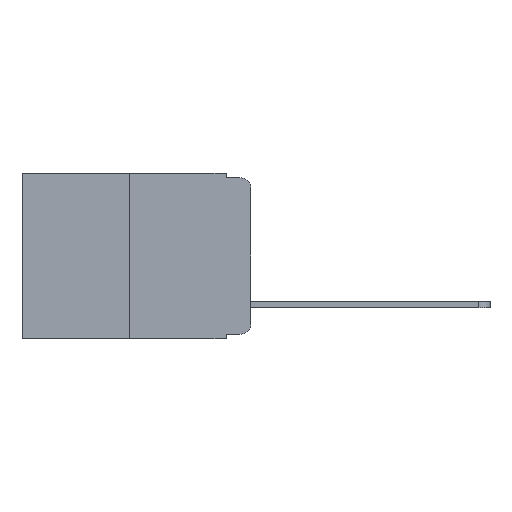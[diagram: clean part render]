
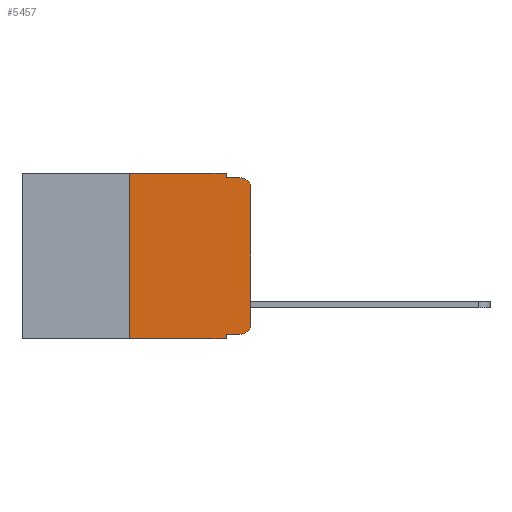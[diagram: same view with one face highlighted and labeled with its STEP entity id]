
A CAD part, left-side view. The second image highlights one B-rep face of the part: STEP entity #5457.
In plain terms, the highlighted planar face has unit normal (-1, 0, 0).
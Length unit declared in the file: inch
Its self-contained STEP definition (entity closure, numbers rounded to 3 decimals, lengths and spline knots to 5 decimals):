
#1 = VERTEX_POINT ( 'NONE', #9375 ) ;
#126 = DIRECTION ( 'NONE',  ( 0., 0., -1. ) ) ;
#350 = ORIENTED_EDGE ( 'NONE', *, *, #6454, .F. ) ;
#742 = VERTEX_POINT ( 'NONE', #3904 ) ;
#983 = DIRECTION ( 'NONE',  ( 0., 0., 1. ) ) ;
#1286 = ORIENTED_EDGE ( 'NONE', *, *, #6357, .T. ) ;
#1428 = DIRECTION ( 'NONE',  ( 0., 0., -1. ) ) ;
#1685 = LINE ( 'NONE', #3906, #8695 ) ;
#1980 = LINE ( 'NONE', #2163, #4214 ) ;
#2163 = CARTESIAN_POINT ( 'NONE',  ( 0., 0.051, -0.01 ) ) ;
#2404 = DIRECTION ( 'NONE',  ( 1., 0., 0. ) ) ;
#2427 = ORIENTED_EDGE ( 'NONE', *, *, #2499, .F. ) ;
#2429 = EDGE_CURVE ( 'NONE', #742, #3258, #10871, .T. ) ;
#2499 = EDGE_CURVE ( 'NONE', #16361, #14265, #15868, .T. ) ;
#2777 = VECTOR ( 'NONE', #983, 39.37008 ) ;
#3258 = VERTEX_POINT ( 'NONE', #6796 ) ;
#3377 = EDGE_CURVE ( 'NONE', #7624, #3258, #1980, .T. ) ;
#3547 = LINE ( 'NONE', #13163, #12404 ) ;
#3613 = AXIS2_PLACEMENT_3D ( 'NONE', #10280, #2404, #11426 ) ;
#3671 = PLANE ( 'NONE',  #3613 ) ;
#3904 = CARTESIAN_POINT ( 'NONE',  ( 0., 0., -0.03 ) ) ;
#3906 = CARTESIAN_POINT ( 'NONE',  ( 0., 0.25, 0. ) ) ;
#4214 = VECTOR ( 'NONE', #8501, 39.37008 ) ;
#4229 = FACE_OUTER_BOUND ( 'NONE', #7039, .T. ) ;
#4566 = CARTESIAN_POINT ( 'NONE',  ( 0., 0.02, -0.333 ) ) ;
#4628 = DIRECTION ( 'NONE',  ( 0., -1., 0. ) ) ;
#4681 = CARTESIAN_POINT ( 'NONE',  ( 0., 0.473, -0.343 ) ) ;
#4726 = ORIENTED_EDGE ( 'NONE', *, *, #2429, .T. ) ;
#5040 = CARTESIAN_POINT ( 'NONE',  ( 0., 0.051, -0.01 ) ) ;
#5067 = EDGE_CURVE ( 'NONE', #11892, #5694, #12056, .T. ) ;
#5214 = VECTOR ( 'NONE', #5925, 39.37008 ) ;
#5268 = CARTESIAN_POINT ( 'NONE',  ( 0., 0.02, -0.313 ) ) ;
#5391 = CARTESIAN_POINT ( 'NONE',  ( 0., 0.051, -0.333 ) ) ;
#5457 = ADVANCED_FACE ( 'NONE', ( #4229 ), #3671, .F. ) ;
#5694 = VERTEX_POINT ( 'NONE', #8194 ) ;
#5756 = VERTEX_POINT ( 'NONE', #7447 ) ;
#5925 = DIRECTION ( 'NONE',  ( 0., -1., 0. ) ) ;
#6032 = ORIENTED_EDGE ( 'NONE', *, *, #7830, .T. ) ;
#6115 = ORIENTED_EDGE ( 'NONE', *, *, #3377, .F. ) ;
#6357 = EDGE_CURVE ( 'NONE', #1, #14265, #7944, .T. ) ;
#6454 = EDGE_CURVE ( 'NONE', #5694, #7624, #3547, .T. ) ;
#6521 = DIRECTION ( 'NONE',  ( -1., 0., 0. ) ) ;
#6796 = CARTESIAN_POINT ( 'NONE',  ( 0., 0.02, -0.01 ) ) ;
#7039 = EDGE_LOOP ( 'NONE', ( #10311, #4726, #6115, #350, #8776, #14311, #1286, #2427, #14214, #6032 ) ) ;
#7447 = CARTESIAN_POINT ( 'NONE',  ( 0., 0., -0.313 ) ) ;
#7624 = VERTEX_POINT ( 'NONE', #5040 ) ;
#7830 = EDGE_CURVE ( 'NONE', #15564, #5756, #10654, .T. ) ;
#7921 = DIRECTION ( 'NONE',  ( 0., 0., -1. ) ) ;
#7944 = LINE ( 'NONE', #4681, #12189 ) ;
#8194 = CARTESIAN_POINT ( 'NONE',  ( 0., 0.051, 0. ) ) ;
#8211 = CARTESIAN_POINT ( 'NONE',  ( 0., 0.473, 0. ) ) ;
#8479 = EDGE_CURVE ( 'NONE', #16361, #15564, #16590, .T. ) ;
#8501 = DIRECTION ( 'NONE',  ( 0., -1., 0. ) ) ;
#8619 = VECTOR ( 'NONE', #7921, 39.37008 ) ;
#8695 = VECTOR ( 'NONE', #16495, 39.37008 ) ;
#8776 = ORIENTED_EDGE ( 'NONE', *, *, #5067, .F. ) ;
#9102 = CARTESIAN_POINT ( 'NONE',  ( 0., 0.051, -0.333 ) ) ;
#9375 = CARTESIAN_POINT ( 'NONE',  ( 0., 0.25, -0.343 ) ) ;
#10276 = CARTESIAN_POINT ( 'NONE',  ( 0., 0.25, 0. ) ) ;
#10280 = CARTESIAN_POINT ( 'NONE',  ( 0., 0.473, 0. ) ) ;
#10311 = ORIENTED_EDGE ( 'NONE', *, *, #12429, .T. ) ;
#10590 = CARTESIAN_POINT ( 'NONE',  ( 0., 0.051, 0. ) ) ;
#10654 = CIRCLE ( 'NONE', #14746, 0.02 ) ;
#10871 = CIRCLE ( 'NONE', #12774, 0.02 ) ;
#10958 = CARTESIAN_POINT ( 'NONE',  ( 0., 0.051, -0.343 ) ) ;
#11236 = LINE ( 'NONE', #15024, #2777 ) ;
#11426 = DIRECTION ( 'NONE',  ( 0., 0., -1. ) ) ;
#11892 = VERTEX_POINT ( 'NONE', #10276 ) ;
#12056 = LINE ( 'NONE', #8211, #5214 ) ;
#12189 = VECTOR ( 'NONE', #4628, 39.37008 ) ;
#12404 = VECTOR ( 'NONE', #13114, 39.37008 ) ;
#12429 = EDGE_CURVE ( 'NONE', #5756, #742, #11236, .T. ) ;
#12774 = AXIS2_PLACEMENT_3D ( 'NONE', #14254, #6521, #1428 ) ;
#13114 = DIRECTION ( 'NONE',  ( 0., 0., -1. ) ) ;
#13126 = DIRECTION ( 'NONE',  ( 0., -1., 0. ) ) ;
#13163 = CARTESIAN_POINT ( 'NONE',  ( 0., 0.051, 0. ) ) ;
#14211 = DIRECTION ( 'NONE',  ( -1., 0., 0. ) ) ;
#14214 = ORIENTED_EDGE ( 'NONE', *, *, #8479, .T. ) ;
#14254 = CARTESIAN_POINT ( 'NONE',  ( 0., 0.02, -0.03 ) ) ;
#14265 = VERTEX_POINT ( 'NONE', #10958 ) ;
#14311 = ORIENTED_EDGE ( 'NONE', *, *, #14973, .F. ) ;
#14746 = AXIS2_PLACEMENT_3D ( 'NONE', #5268, #14211, #126 ) ;
#14973 = EDGE_CURVE ( 'NONE', #1, #11892, #1685, .T. ) ;
#15024 = CARTESIAN_POINT ( 'NONE',  ( 0., 0., 0. ) ) ;
#15564 = VERTEX_POINT ( 'NONE', #4566 ) ;
#15868 = LINE ( 'NONE', #10590, #8619 ) ;
#16216 = VECTOR ( 'NONE', #13126, 39.37008 ) ;
#16361 = VERTEX_POINT ( 'NONE', #9102 ) ;
#16495 = DIRECTION ( 'NONE',  ( 0., 0., 1. ) ) ;
#16590 = LINE ( 'NONE', #5391, #16216 ) ;
